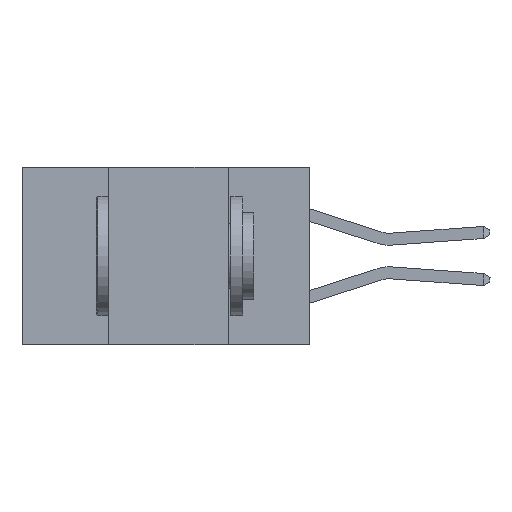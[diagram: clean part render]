
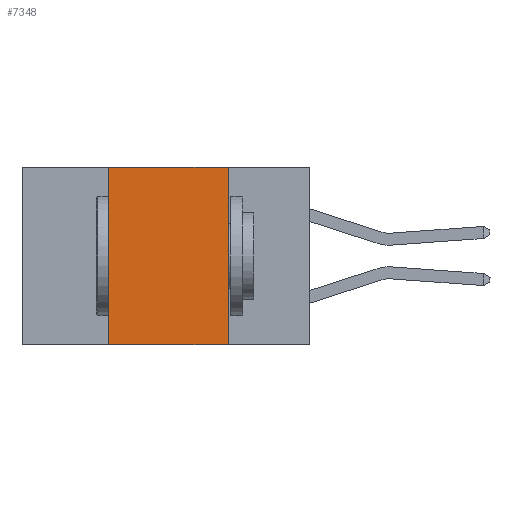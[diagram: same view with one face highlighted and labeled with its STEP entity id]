
A CAD part, left-side view. The second image highlights one B-rep face of the part: STEP entity #7348.
In plain terms, the highlighted planar face has unit normal (-1, 0, 0).
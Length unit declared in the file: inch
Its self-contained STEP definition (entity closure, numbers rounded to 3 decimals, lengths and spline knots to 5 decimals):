
#1351 = CARTESIAN_POINT ( 'NONE',  ( 0., 0.42, -0.37 ) ) ;
#1553 = EDGE_CURVE ( 'NONE', #2655, #14540, #8084, .T. ) ;
#2229 = ORIENTED_EDGE ( 'NONE', *, *, #7306, .F. ) ;
#2264 = ORIENTED_EDGE ( 'NONE', *, *, #8913, .F. ) ;
#2342 = VECTOR ( 'NONE', #16164, 39.37008 ) ;
#2535 = DIRECTION ( 'NONE',  ( 0., -1., 0. ) ) ;
#2651 = ORIENTED_EDGE ( 'NONE', *, *, #1553, .F. ) ;
#2655 = VERTEX_POINT ( 'NONE', #1351 ) ;
#2786 = CARTESIAN_POINT ( 'NONE',  ( 0., 0.6, 0. ) ) ;
#2938 = ORIENTED_EDGE ( 'NONE', *, *, #7386, .T. ) ;
#3204 = CARTESIAN_POINT ( 'NONE',  ( 0., 0.42, 0. ) ) ;
#4930 = LINE ( 'NONE', #16221, #15781 ) ;
#6060 = DIRECTION ( 'NONE',  ( 0., 0., 1. ) ) ;
#7280 = VERTEX_POINT ( 'NONE', #16592 ) ;
#7306 = EDGE_CURVE ( 'NONE', #7280, #16432, #10045, .T. ) ;
#7348 = ADVANCED_FACE ( 'NONE', ( #16685 ), #15882, .F. ) ;
#7386 = EDGE_CURVE ( 'NONE', #2655, #16432, #4930, .T. ) ;
#7815 = EDGE_LOOP ( 'NONE', ( #2229, #2264, #2651, #2938 ) ) ;
#8084 = LINE ( 'NONE', #3204, #11410 ) ;
#8422 = CARTESIAN_POINT ( 'NONE',  ( 0., 0.42, 0. ) ) ;
#8913 = EDGE_CURVE ( 'NONE', #14540, #7280, #16402, .T. ) ;
#10045 = LINE ( 'NONE', #16232, #2342 ) ;
#11410 = VECTOR ( 'NONE', #6060, 39.37008 ) ;
#12451 = VECTOR ( 'NONE', #2535, 39.37008 ) ;
#14540 = VERTEX_POINT ( 'NONE', #8422 ) ;
#15058 = AXIS2_PLACEMENT_3D ( 'NONE', #16023, #15859, #15856 ) ;
#15481 = DIRECTION ( 'NONE',  ( 0., -1., 0. ) ) ;
#15781 = VECTOR ( 'NONE', #15481, 39.37008 ) ;
#15856 = DIRECTION ( 'NONE',  ( 0., 0., -1. ) ) ;
#15859 = DIRECTION ( 'NONE',  ( 1., 0., 0. ) ) ;
#15880 = CARTESIAN_POINT ( 'NONE',  ( 0., 0.17, -0.37 ) ) ;
#15882 = PLANE ( 'NONE',  #15058 ) ;
#16023 = CARTESIAN_POINT ( 'NONE',  ( 0., 0.6, 0. ) ) ;
#16164 = DIRECTION ( 'NONE',  ( 0., 0., -1. ) ) ;
#16221 = CARTESIAN_POINT ( 'NONE',  ( 0., 0.6, -0.37 ) ) ;
#16232 = CARTESIAN_POINT ( 'NONE',  ( 0., 0.17, 0. ) ) ;
#16402 = LINE ( 'NONE', #2786, #12451 ) ;
#16432 = VERTEX_POINT ( 'NONE', #15880 ) ;
#16592 = CARTESIAN_POINT ( 'NONE',  ( 0., 0.17, 0. ) ) ;
#16685 = FACE_OUTER_BOUND ( 'NONE', #7815, .T. ) ;
